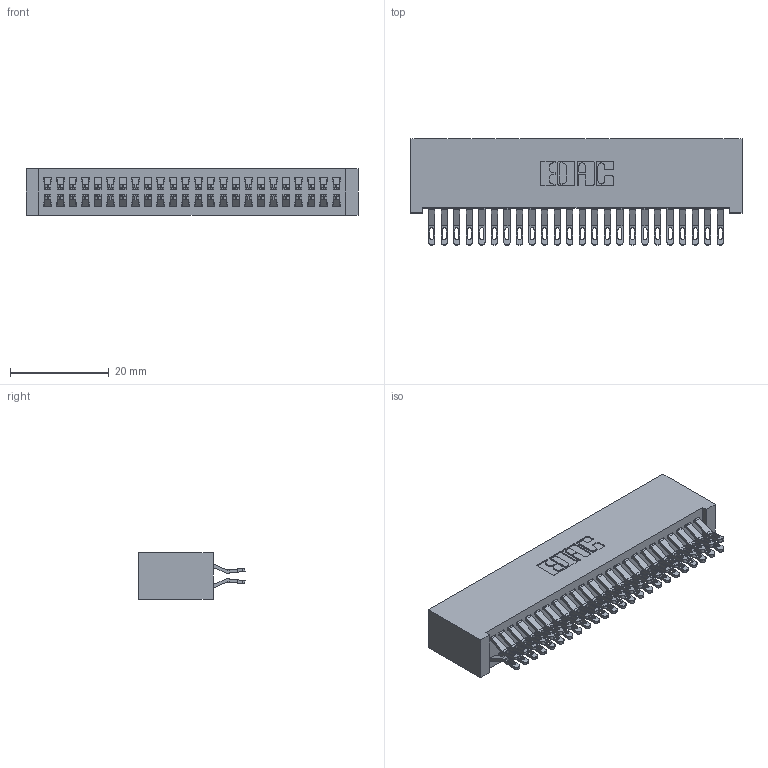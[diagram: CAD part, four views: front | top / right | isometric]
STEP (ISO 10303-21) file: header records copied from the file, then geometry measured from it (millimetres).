
FILE_DESCRIPTION (( 'STEP AP203' ), '1' );
FILE_NAME ('342-048-555-201.STEP', '2018-08-12T18:16:59', ( '' ), ( '' ), 'SwSTEP 2.0', 'SolidWorks 2016', '' );
FILE_SCHEMA (( 'CONFIG_CONTROL_DESIGN' ));
Length unit declared in the file: inch
Products named in the file (3): 342 Part_Lugless; 345-292-001_555 Tail; 342-048-555-201
Assembly tree (49 placements, depth 2):
  342-048-555-201
    342 Part_Lugless
    345-292-001_555 Tail  x48
Bounding box: 67.21 x 21.47 x 9.4 mm (x, y, z)
Volume: 6526.4 mm3; surface area: 11090.4 mm2
Topology: 49 solids, 49 shells, 2886 faces, 9059 edges, 6038 vertices
Faces by surface type: plane 1694, cylinder 1192
Entity records: 17685 total; most frequent: CARTESIAN_POINT 2984, ORIENTED_EDGE 2890, DIRECTION 2545, EDGE_CURVE 1445, LINE 1305, VECTOR 1305, VERTEX_POINT 962, AXIS2_PLACEMENT_3D 620
